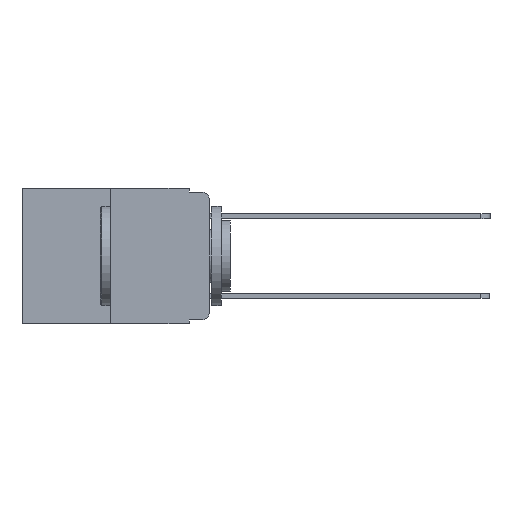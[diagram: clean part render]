
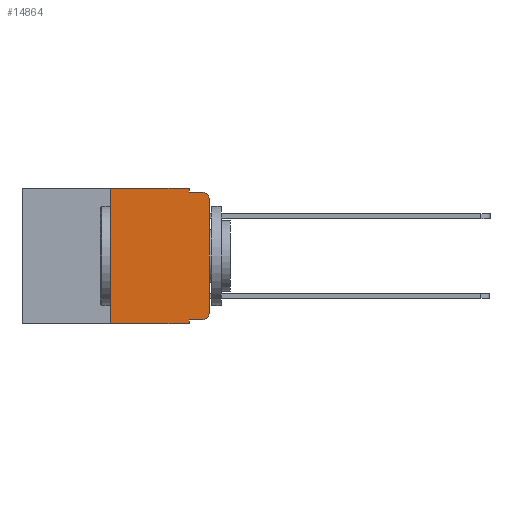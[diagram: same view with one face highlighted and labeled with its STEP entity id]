
A CAD part, left-side view. The second image highlights one B-rep face of the part: STEP entity #14864.
In plain terms, the highlighted planar face has unit normal (-1, 0, 0).
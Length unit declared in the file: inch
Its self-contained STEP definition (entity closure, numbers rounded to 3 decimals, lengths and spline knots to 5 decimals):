
#184 = EDGE_CURVE ( 'NONE', #6584, #5887, #16060, .T. ) ;
#477 = EDGE_CURVE ( 'NONE', #5887, #1507, #5938, .T. ) ;
#658 = LINE ( 'NONE', #21015, #15099 ) ;
#686 = CARTESIAN_POINT ( 'NONE',  ( 0., 0.02, -0.01 ) ) ;
#1022 = EDGE_CURVE ( 'NONE', #20615, #1507, #7282, .T. ) ;
#1167 = VECTOR ( 'NONE', #7231, 39.37008 ) ;
#1169 = ORIENTED_EDGE ( 'NONE', *, *, #13898, .T. ) ;
#1224 = EDGE_CURVE ( 'NONE', #10189, #20217, #12754, .T. ) ;
#1272 = CARTESIAN_POINT ( 'NONE',  ( 0., 0.051, -0.01 ) ) ;
#1443 = EDGE_LOOP ( 'NONE', ( #1169, #7744, #9159, #2333, #17082, #19370, #4391, #7120, #5242, #3351 ) ) ;
#1507 = VERTEX_POINT ( 'NONE', #686 ) ;
#1714 = DIRECTION ( 'NONE',  ( 0., 0., 1. ) ) ;
#2069 = CARTESIAN_POINT ( 'NONE',  ( 0., 0.051, -0.343 ) ) ;
#2333 = ORIENTED_EDGE ( 'NONE', *, *, #184, .F. ) ;
#2708 = EDGE_CURVE ( 'NONE', #3265, #6584, #658, .T. ) ;
#2986 = CARTESIAN_POINT ( 'NONE',  ( 0., 0.02, -0.03 ) ) ;
#3065 = DIRECTION ( 'NONE',  ( -1., 0., 0. ) ) ;
#3265 = VERTEX_POINT ( 'NONE', #20911 ) ;
#3351 = ORIENTED_EDGE ( 'NONE', *, *, #13504, .T. ) ;
#3759 = DIRECTION ( 'NONE',  ( -1., 0., 0. ) ) ;
#3821 = CARTESIAN_POINT ( 'NONE',  ( 0., 0., -0.313 ) ) ;
#4391 = ORIENTED_EDGE ( 'NONE', *, *, #18604, .T. ) ;
#4562 = DIRECTION ( 'NONE',  ( 0., -1., 0. ) ) ;
#5242 = ORIENTED_EDGE ( 'NONE', *, *, #20126, .T. ) ;
#5759 = LINE ( 'NONE', #12282, #10385 ) ;
#5887 = VERTEX_POINT ( 'NONE', #19987 ) ;
#5938 = LINE ( 'NONE', #1272, #18809 ) ;
#6081 = PLANE ( 'NONE',  #9482 ) ;
#6087 = LINE ( 'NONE', #9822, #10181 ) ;
#6584 = VERTEX_POINT ( 'NONE', #15737 ) ;
#7120 = ORIENTED_EDGE ( 'NONE', *, *, #1224, .F. ) ;
#7231 = DIRECTION ( 'NONE',  ( 0., 0., 1. ) ) ;
#7282 = CIRCLE ( 'NONE', #16755, 0.02 ) ;
#7544 = VECTOR ( 'NONE', #20070, 39.37008 ) ;
#7744 = ORIENTED_EDGE ( 'NONE', *, *, #1022, .T. ) ;
#7761 = VERTEX_POINT ( 'NONE', #14033 ) ;
#8795 = DIRECTION ( 'NONE',  ( 0., 0., -1. ) ) ;
#9159 = ORIENTED_EDGE ( 'NONE', *, *, #477, .F. ) ;
#9482 = AXIS2_PLACEMENT_3D ( 'NONE', #9601, #21855, #11351 ) ;
#9601 = CARTESIAN_POINT ( 'NONE',  ( 0., 0.473, 0. ) ) ;
#9822 = CARTESIAN_POINT ( 'NONE',  ( 0., 0.473, -0.343 ) ) ;
#10181 = VECTOR ( 'NONE', #4562, 39.37008 ) ;
#10189 = VERTEX_POINT ( 'NONE', #15225 ) ;
#10317 = DIRECTION ( 'NONE',  ( 0., 0., -1. ) ) ;
#10385 = VECTOR ( 'NONE', #14040, 39.37008 ) ;
#10447 = EDGE_CURVE ( 'NONE', #16116, #3265, #19791, .T. ) ;
#11351 = DIRECTION ( 'NONE',  ( 0., 0., -1. ) ) ;
#11409 = VECTOR ( 'NONE', #10317, 39.37008 ) ;
#12076 = VECTOR ( 'NONE', #1714, 39.37008 ) ;
#12083 = CARTESIAN_POINT ( 'NONE',  ( 0., 0.051, 0. ) ) ;
#12098 = CIRCLE ( 'NONE', #14004, 0.02 ) ;
#12171 = CARTESIAN_POINT ( 'NONE',  ( 0., 0., 0. ) ) ;
#12282 = CARTESIAN_POINT ( 'NONE',  ( 0., 0.051, -0.333 ) ) ;
#12754 = LINE ( 'NONE', #22121, #7544 ) ;
#13504 = EDGE_CURVE ( 'NONE', #7761, #20219, #12098, .T. ) ;
#13898 = EDGE_CURVE ( 'NONE', #20219, #20615, #21944, .T. ) ;
#14004 = AXIS2_PLACEMENT_3D ( 'NONE', #14204, #3759, #15942 ) ;
#14033 = CARTESIAN_POINT ( 'NONE',  ( 0., 0.02, -0.333 ) ) ;
#14040 = DIRECTION ( 'NONE',  ( 0., -1., 0. ) ) ;
#14204 = CARTESIAN_POINT ( 'NONE',  ( 0., 0.02, -0.313 ) ) ;
#14491 = FACE_OUTER_BOUND ( 'NONE', #1443, .T. ) ;
#14864 = ADVANCED_FACE ( 'NONE', ( #14491 ), #6081, .F. ) ;
#15099 = VECTOR ( 'NONE', #18205, 39.37008 ) ;
#15225 = CARTESIAN_POINT ( 'NONE',  ( 0., 0.051, -0.333 ) ) ;
#15612 = DIRECTION ( 'NONE',  ( 0., -1., 0. ) ) ;
#15737 = CARTESIAN_POINT ( 'NONE',  ( 0., 0.051, 0. ) ) ;
#15942 = DIRECTION ( 'NONE',  ( 0., 0., -1. ) ) ;
#16034 = CARTESIAN_POINT ( 'NONE',  ( 0., 0.25, -0.343 ) ) ;
#16060 = LINE ( 'NONE', #12083, #11409 ) ;
#16116 = VERTEX_POINT ( 'NONE', #16034 ) ;
#16755 = AXIS2_PLACEMENT_3D ( 'NONE', #2986, #3065, #8795 ) ;
#17082 = ORIENTED_EDGE ( 'NONE', *, *, #2708, .F. ) ;
#18205 = DIRECTION ( 'NONE',  ( 0., -1., 0. ) ) ;
#18604 = EDGE_CURVE ( 'NONE', #16116, #20217, #6087, .T. ) ;
#18809 = VECTOR ( 'NONE', #15612, 39.37008 ) ;
#19370 = ORIENTED_EDGE ( 'NONE', *, *, #10447, .F. ) ;
#19487 = CARTESIAN_POINT ( 'NONE',  ( 0., 0.25, 0. ) ) ;
#19791 = LINE ( 'NONE', #19487, #1167 ) ;
#19987 = CARTESIAN_POINT ( 'NONE',  ( 0., 0.051, -0.01 ) ) ;
#20070 = DIRECTION ( 'NONE',  ( 0., 0., -1. ) ) ;
#20126 = EDGE_CURVE ( 'NONE', #10189, #7761, #5759, .T. ) ;
#20217 = VERTEX_POINT ( 'NONE', #2069 ) ;
#20219 = VERTEX_POINT ( 'NONE', #3821 ) ;
#20615 = VERTEX_POINT ( 'NONE', #22606 ) ;
#20911 = CARTESIAN_POINT ( 'NONE',  ( 0., 0.25, 0. ) ) ;
#21015 = CARTESIAN_POINT ( 'NONE',  ( 0., 0.473, 0. ) ) ;
#21855 = DIRECTION ( 'NONE',  ( 1., 0., 0. ) ) ;
#21944 = LINE ( 'NONE', #12171, #12076 ) ;
#22121 = CARTESIAN_POINT ( 'NONE',  ( 0., 0.051, 0. ) ) ;
#22606 = CARTESIAN_POINT ( 'NONE',  ( 0., 0., -0.03 ) ) ;
